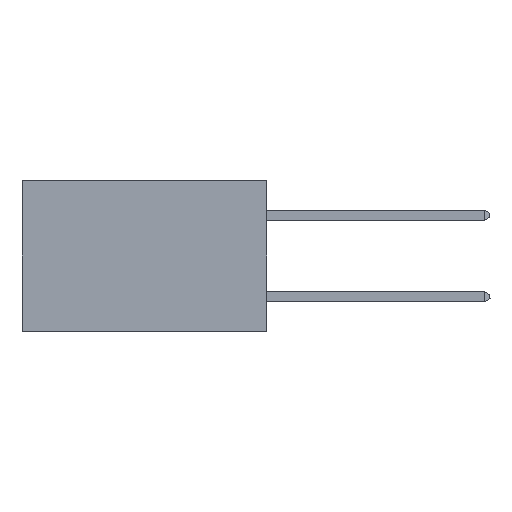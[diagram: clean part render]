
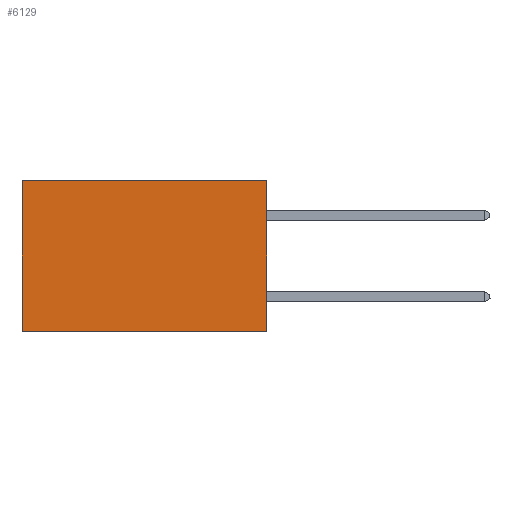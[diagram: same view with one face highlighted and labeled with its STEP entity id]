
A CAD part, left-side view. The second image highlights one B-rep face of the part: STEP entity #6129.
In plain terms, the highlighted planar face has unit normal (-1, 0, 0).
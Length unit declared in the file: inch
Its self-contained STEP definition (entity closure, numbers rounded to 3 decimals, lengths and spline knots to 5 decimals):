
#76 = VERTEX_POINT ( 'NONE', #21686 ) ;
#1614 = EDGE_CURVE ( 'NONE', #76, #13591, #12810, .T. ) ;
#1714 = PLANE ( 'NONE',  #8205 ) ;
#2170 = DIRECTION ( 'NONE',  ( 0., 1., 0. ) ) ;
#3115 = ORIENTED_EDGE ( 'NONE', *, *, #1614, .F. ) ;
#4964 = VECTOR ( 'NONE', #21948, 39.37008 ) ;
#5101 = DIRECTION ( 'NONE',  ( 0., 0., -1. ) ) ;
#6129 = ADVANCED_FACE ( 'NONE', ( #9884 ), #1714, .F. ) ;
#6181 = CARTESIAN_POINT ( 'NONE',  ( 0.2875, 0., 0. ) ) ;
#6922 = VECTOR ( 'NONE', #24459, 39.37008 ) ;
#7004 = CARTESIAN_POINT ( 'NONE',  ( 0.2875, 0., 0. ) ) ;
#8205 = AXIS2_PLACEMENT_3D ( 'NONE', #6181, #21464, #8427 ) ;
#8427 = DIRECTION ( 'NONE',  ( 0., 0., -1. ) ) ;
#8726 = VECTOR ( 'NONE', #5101, 39.37008 ) ;
#9884 = FACE_OUTER_BOUND ( 'NONE', #17337, .T. ) ;
#12810 = LINE ( 'NONE', #7004, #6922 ) ;
#12888 = ORIENTED_EDGE ( 'NONE', *, *, #26084, .T. ) ;
#13591 = VERTEX_POINT ( 'NONE', #14206 ) ;
#14206 = CARTESIAN_POINT ( 'NONE',  ( 0.2875, 0., -0.37 ) ) ;
#15422 = CARTESIAN_POINT ( 'NONE',  ( 0.2875, 0., -0.37 ) ) ;
#16764 = EDGE_CURVE ( 'NONE', #13591, #26829, #26021, .T. ) ;
#17337 = EDGE_LOOP ( 'NONE', ( #22201, #26850, #3115, #12888 ) ) ;
#18629 = CARTESIAN_POINT ( 'NONE',  ( 0.2875, 0.6, -0.37 ) ) ;
#19765 = CARTESIAN_POINT ( 'NONE',  ( 0.2875, 0., 0. ) ) ;
#20586 = VERTEX_POINT ( 'NONE', #23691 ) ;
#21010 = VECTOR ( 'NONE', #2170, 39.37008 ) ;
#21464 = DIRECTION ( 'NONE',  ( 1., 0., 0. ) ) ;
#21686 = CARTESIAN_POINT ( 'NONE',  ( 0.2875, 0., 0. ) ) ;
#21948 = DIRECTION ( 'NONE',  ( 0., 1., 0. ) ) ;
#22201 = ORIENTED_EDGE ( 'NONE', *, *, #28038, .T. ) ;
#22440 = LINE ( 'NONE', #19765, #4964 ) ;
#23029 = LINE ( 'NONE', #24788, #8726 ) ;
#23691 = CARTESIAN_POINT ( 'NONE',  ( 0.2875, 0.6, 0. ) ) ;
#24459 = DIRECTION ( 'NONE',  ( 0., 0., -1. ) ) ;
#24788 = CARTESIAN_POINT ( 'NONE',  ( 0.2875, 0.6, 0. ) ) ;
#26021 = LINE ( 'NONE', #15422, #21010 ) ;
#26084 = EDGE_CURVE ( 'NONE', #76, #20586, #22440, .T. ) ;
#26829 = VERTEX_POINT ( 'NONE', #18629 ) ;
#26850 = ORIENTED_EDGE ( 'NONE', *, *, #16764, .F. ) ;
#28038 = EDGE_CURVE ( 'NONE', #20586, #26829, #23029, .T. ) ;
